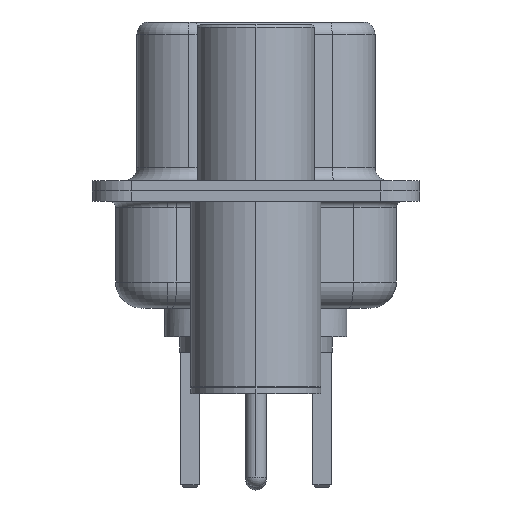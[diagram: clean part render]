
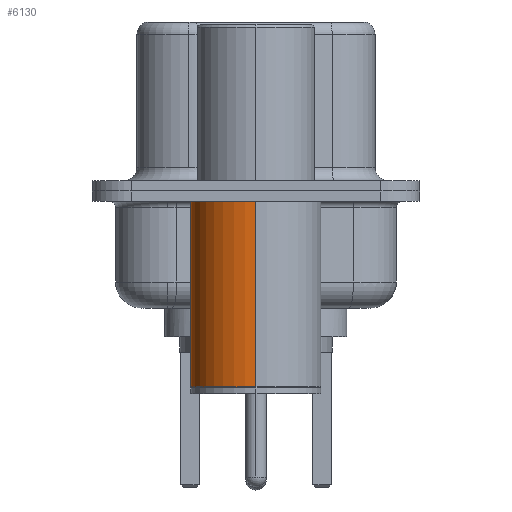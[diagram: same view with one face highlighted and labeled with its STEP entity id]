
A CAD part, left-side view. The second image highlights one B-rep face of the part: STEP entity #6130.
In plain terms, the highlighted cylindrical face has radius 2.5 mm (diameter 5 mm), a partial arc.
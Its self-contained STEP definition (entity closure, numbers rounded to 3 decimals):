
#870 = EDGE_CURVE ( 'NONE', #4187, #25172, #22188, .T. ) ;
#2408 = CARTESIAN_POINT ( 'NONE',  ( 2.5, 0., 0.581 ) ) ;
#3113 = CARTESIAN_POINT ( 'NONE',  ( -2.5, 0., 0.581 ) ) ;
#3284 = AXIS2_PLACEMENT_3D ( 'NONE', #19895, #7522, #21970 ) ;
#3671 = EDGE_CURVE ( 'NONE', #5450, #21164, #6602, .T. ) ;
#3763 = EDGE_CURVE ( 'NONE', #5450, #4187, #4680, .T. ) ;
#4187 = VERTEX_POINT ( 'NONE', #6400 ) ;
#4517 = DIRECTION ( 'NONE',  ( 1., 0., 0. ) ) ;
#4680 = CIRCLE ( 'NONE', #8637, 2.5 ) ;
#4763 = ORIENTED_EDGE ( 'NONE', *, *, #3671, .F. ) ;
#5450 = VERTEX_POINT ( 'NONE', #24591 ) ;
#5781 = ORIENTED_EDGE ( 'NONE', *, *, #25516, .F. ) ;
#5896 = CARTESIAN_POINT ( 'NONE',  ( -2.5, 0., -0.4 ) ) ;
#6130 = ADVANCED_FACE ( 'NONE', ( #11713 ), #26148, .T. ) ;
#6400 = CARTESIAN_POINT ( 'NONE',  ( -2.5, 0., -7.525 ) ) ;
#6602 = LINE ( 'NONE', #2408, #11474 ) ;
#7522 = DIRECTION ( 'NONE',  ( 0., 0., 1. ) ) ;
#8637 = AXIS2_PLACEMENT_3D ( 'NONE', #26103, #26021, #25844 ) ;
#9811 = ORIENTED_EDGE ( 'NONE', *, *, #3763, .T. ) ;
#10298 = DIRECTION ( 'NONE',  ( 0., 0., 1. ) ) ;
#11474 = VECTOR ( 'NONE', #26308, 1000. ) ;
#11713 = FACE_OUTER_BOUND ( 'NONE', #22883, .T. ) ;
#12560 = VECTOR ( 'NONE', #18950, 1000. ) ;
#15077 = AXIS2_PLACEMENT_3D ( 'NONE', #20547, #10298, #4517 ) ;
#16930 = CIRCLE ( 'NONE', #3284, 2.5 ) ;
#17080 = ORIENTED_EDGE ( 'NONE', *, *, #870, .T. ) ;
#18950 = DIRECTION ( 'NONE',  ( 0., 0., 1. ) ) ;
#19099 = CARTESIAN_POINT ( 'NONE',  ( 2.5, 0., -0.4 ) ) ;
#19895 = CARTESIAN_POINT ( 'NONE',  ( 0., 0., -0.4 ) ) ;
#20547 = CARTESIAN_POINT ( 'NONE',  ( 0., 0., 0.581 ) ) ;
#21164 = VERTEX_POINT ( 'NONE', #19099 ) ;
#21970 = DIRECTION ( 'NONE',  ( 1., 0., 0. ) ) ;
#22188 = LINE ( 'NONE', #3113, #12560 ) ;
#22883 = EDGE_LOOP ( 'NONE', ( #9811, #17080, #5781, #4763 ) ) ;
#24591 = CARTESIAN_POINT ( 'NONE',  ( 2.5, 0., -7.525 ) ) ;
#25172 = VERTEX_POINT ( 'NONE', #5896 ) ;
#25516 = EDGE_CURVE ( 'NONE', #21164, #25172, #16930, .T. ) ;
#25844 = DIRECTION ( 'NONE',  ( 1., 0., 0. ) ) ;
#26021 = DIRECTION ( 'NONE',  ( 0., 0., 1. ) ) ;
#26103 = CARTESIAN_POINT ( 'NONE',  ( 0., 0., -7.525 ) ) ;
#26148 = CYLINDRICAL_SURFACE ( 'NONE', #15077, 2.5 ) ;
#26308 = DIRECTION ( 'NONE',  ( 0., 0., 1. ) ) ;
